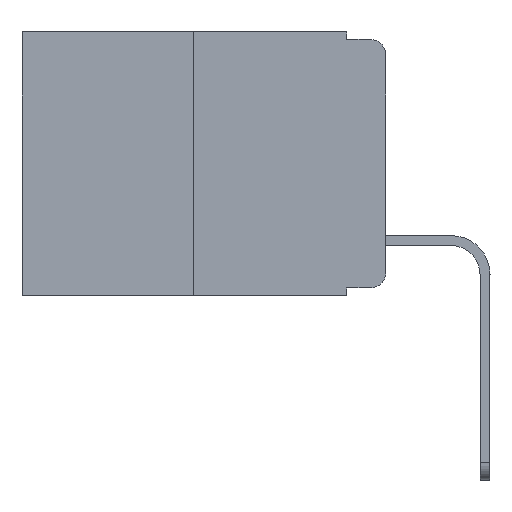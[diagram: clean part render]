
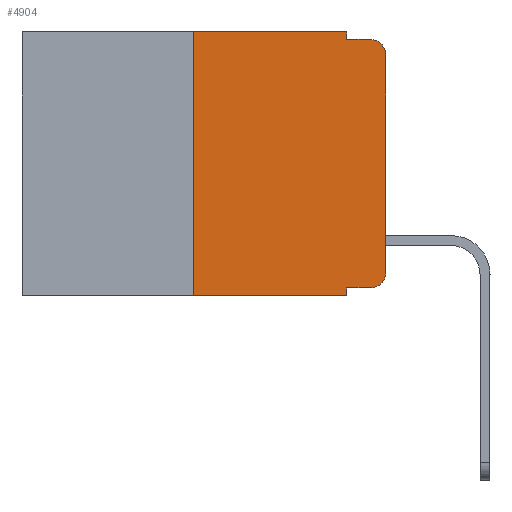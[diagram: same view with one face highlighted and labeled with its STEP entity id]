
A CAD part, left-side view. The second image highlights one B-rep face of the part: STEP entity #4904.
In plain terms, the highlighted planar face has unit normal (-1, 0, 0).
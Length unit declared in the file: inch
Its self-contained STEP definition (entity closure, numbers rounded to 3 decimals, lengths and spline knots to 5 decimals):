
#111 = EDGE_CURVE ( 'NONE', #425, #3170, #468, .T. ) ;
#115 = VECTOR ( 'NONE', #6191, 39.37008 ) ;
#331 = EDGE_CURVE ( 'NONE', #7604, #6732, #9214, .T. ) ;
#425 = VERTEX_POINT ( 'NONE', #9317 ) ;
#468 = LINE ( 'NONE', #1195, #6391 ) ;
#666 = CARTESIAN_POINT ( 'NONE',  ( 0., 0.051, 0. ) ) ;
#1180 = LINE ( 'NONE', #5102, #4402 ) ;
#1181 = DIRECTION ( 'NONE',  ( 0., 0., -1. ) ) ;
#1195 = CARTESIAN_POINT ( 'NONE',  ( 0., 0.473, 0. ) ) ;
#1221 = DIRECTION ( 'NONE',  ( -1., 0., 0. ) ) ;
#1292 = CARTESIAN_POINT ( 'NONE',  ( 0., 0., -0.313 ) ) ;
#1466 = DIRECTION ( 'NONE',  ( 0., -1., 0. ) ) ;
#1490 = CARTESIAN_POINT ( 'NONE',  ( 0., 0.051, 0. ) ) ;
#1541 = VERTEX_POINT ( 'NONE', #10601 ) ;
#1718 = EDGE_CURVE ( 'NONE', #8805, #1541, #4118, .T. ) ;
#2200 = EDGE_CURVE ( 'NONE', #9071, #1541, #1180, .T. ) ;
#2232 = EDGE_CURVE ( 'NONE', #8805, #3053, #3378, .T. ) ;
#2427 = ORIENTED_EDGE ( 'NONE', *, *, #1718, .F. ) ;
#2429 = EDGE_LOOP ( 'NONE', ( #6731, #11127, #11704, #6107, #3919, #11459, #8963, #2427, #12116, #11560 ) ) ;
#2870 = DIRECTION ( 'NONE',  ( 0., 0., 1. ) ) ;
#3053 = VERTEX_POINT ( 'NONE', #4177 ) ;
#3082 = AXIS2_PLACEMENT_3D ( 'NONE', #10693, #11529, #1181 ) ;
#3088 = CARTESIAN_POINT ( 'NONE',  ( 0., 0., 0. ) ) ;
#3170 = VERTEX_POINT ( 'NONE', #666 ) ;
#3210 = VERTEX_POINT ( 'NONE', #1292 ) ;
#3378 = LINE ( 'NONE', #10623, #9154 ) ;
#3582 = DIRECTION ( 'NONE',  ( 0., 0., -1. ) ) ;
#3919 = ORIENTED_EDGE ( 'NONE', *, *, #111, .F. ) ;
#4040 = FACE_OUTER_BOUND ( 'NONE', #2429, .T. ) ;
#4118 = LINE ( 'NONE', #1490, #115 ) ;
#4122 = EDGE_CURVE ( 'NONE', #3170, #7604, #11788, .T. ) ;
#4177 = CARTESIAN_POINT ( 'NONE',  ( 0., 0.02, -0.333 ) ) ;
#4290 = CIRCLE ( 'NONE', #11262, 0.02 ) ;
#4402 = VECTOR ( 'NONE', #7044, 39.37008 ) ;
#4409 = EDGE_CURVE ( 'NONE', #3210, #11486, #9556, .T. ) ;
#4673 = VECTOR ( 'NONE', #2870, 39.37008 ) ;
#4904 = ADVANCED_FACE ( 'NONE', ( #4040 ), #8824, .F. ) ;
#4936 = DIRECTION ( 'NONE',  ( 0., 0., 1. ) ) ;
#5102 = CARTESIAN_POINT ( 'NONE',  ( 0., 0.473, -0.343 ) ) ;
#5217 = CARTESIAN_POINT ( 'NONE',  ( 0., 0.051, -0.333 ) ) ;
#5747 = DIRECTION ( 'NONE',  ( 0., 0., -1. ) ) ;
#5935 = DIRECTION ( 'NONE',  ( 0., 0., -1. ) ) ;
#5939 = EDGE_CURVE ( 'NONE', #11486, #6732, #4290, .T. ) ;
#5964 = CARTESIAN_POINT ( 'NONE',  ( 0., 0., -0.03 ) ) ;
#6005 = VECTOR ( 'NONE', #4936, 39.37008 ) ;
#6107 = ORIENTED_EDGE ( 'NONE', *, *, #4122, .F. ) ;
#6191 = DIRECTION ( 'NONE',  ( 0., 0., -1. ) ) ;
#6391 = VECTOR ( 'NONE', #8760, 39.37008 ) ;
#6430 = VECTOR ( 'NONE', #3582, 39.37008 ) ;
#6695 = VECTOR ( 'NONE', #1466, 39.37008 ) ;
#6731 = ORIENTED_EDGE ( 'NONE', *, *, #4409, .T. ) ;
#6732 = VERTEX_POINT ( 'NONE', #11580 ) ;
#6748 = CARTESIAN_POINT ( 'NONE',  ( 0., 0.25, 0. ) ) ;
#7042 = LINE ( 'NONE', #6748, #4673 ) ;
#7044 = DIRECTION ( 'NONE',  ( 0., -1., 0. ) ) ;
#7242 = EDGE_CURVE ( 'NONE', #3053, #3210, #11397, .T. ) ;
#7604 = VERTEX_POINT ( 'NONE', #10093 ) ;
#8760 = DIRECTION ( 'NONE',  ( 0., -1., 0. ) ) ;
#8805 = VERTEX_POINT ( 'NONE', #5217 ) ;
#8824 = PLANE ( 'NONE',  #3082 ) ;
#8832 = DIRECTION ( 'NONE',  ( 0., -1., 0. ) ) ;
#8963 = ORIENTED_EDGE ( 'NONE', *, *, #2200, .T. ) ;
#9071 = VERTEX_POINT ( 'NONE', #11351 ) ;
#9154 = VECTOR ( 'NONE', #8832, 39.37008 ) ;
#9214 = LINE ( 'NONE', #10974, #6695 ) ;
#9317 = CARTESIAN_POINT ( 'NONE',  ( 0., 0.25, 0. ) ) ;
#9376 = DIRECTION ( 'NONE',  ( -1., 0., 0. ) ) ;
#9483 = EDGE_CURVE ( 'NONE', #9071, #425, #7042, .T. ) ;
#9556 = LINE ( 'NONE', #3088, #6005 ) ;
#10093 = CARTESIAN_POINT ( 'NONE',  ( 0., 0.051, -0.01 ) ) ;
#10165 = CARTESIAN_POINT ( 'NONE',  ( 0., 0.051, 0. ) ) ;
#10340 = CARTESIAN_POINT ( 'NONE',  ( 0., 0.02, -0.03 ) ) ;
#10601 = CARTESIAN_POINT ( 'NONE',  ( 0., 0.051, -0.343 ) ) ;
#10623 = CARTESIAN_POINT ( 'NONE',  ( 0., 0.051, -0.333 ) ) ;
#10693 = CARTESIAN_POINT ( 'NONE',  ( 0., 0.473, 0. ) ) ;
#10974 = CARTESIAN_POINT ( 'NONE',  ( 0., 0.051, -0.01 ) ) ;
#11127 = ORIENTED_EDGE ( 'NONE', *, *, #5939, .T. ) ;
#11262 = AXIS2_PLACEMENT_3D ( 'NONE', #10340, #9376, #5747 ) ;
#11351 = CARTESIAN_POINT ( 'NONE',  ( 0., 0.25, -0.343 ) ) ;
#11397 = CIRCLE ( 'NONE', #12233, 0.02 ) ;
#11459 = ORIENTED_EDGE ( 'NONE', *, *, #9483, .F. ) ;
#11486 = VERTEX_POINT ( 'NONE', #5964 ) ;
#11529 = DIRECTION ( 'NONE',  ( 1., 0., 0. ) ) ;
#11560 = ORIENTED_EDGE ( 'NONE', *, *, #7242, .T. ) ;
#11567 = CARTESIAN_POINT ( 'NONE',  ( 0., 0.02, -0.313 ) ) ;
#11580 = CARTESIAN_POINT ( 'NONE',  ( 0., 0.02, -0.01 ) ) ;
#11704 = ORIENTED_EDGE ( 'NONE', *, *, #331, .F. ) ;
#11788 = LINE ( 'NONE', #10165, #6430 ) ;
#12116 = ORIENTED_EDGE ( 'NONE', *, *, #2232, .T. ) ;
#12233 = AXIS2_PLACEMENT_3D ( 'NONE', #11567, #1221, #5935 ) ;
